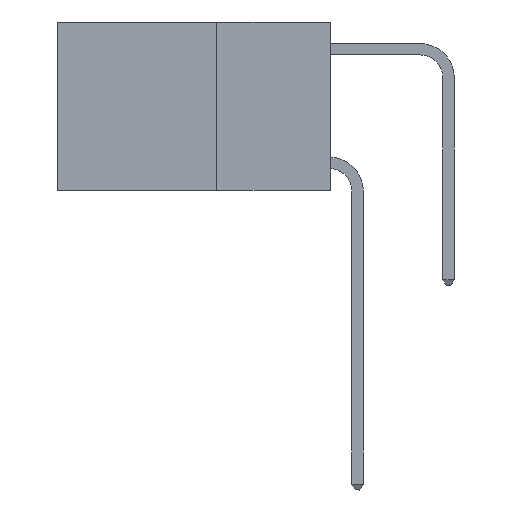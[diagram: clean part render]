
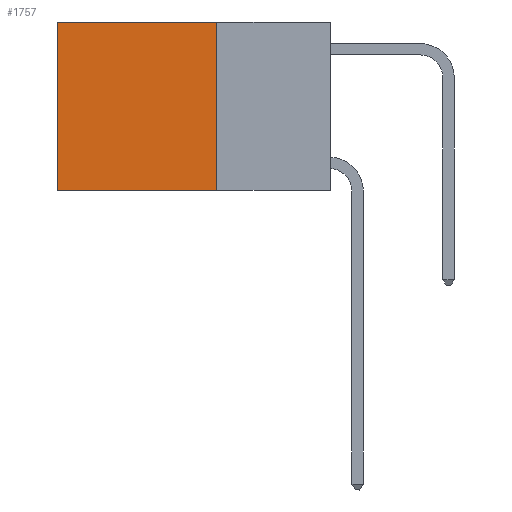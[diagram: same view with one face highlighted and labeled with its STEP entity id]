
A CAD part, left-side view. The second image highlights one B-rep face of the part: STEP entity #1757.
In plain terms, the highlighted planar face has unit normal (-1, 0, 0).
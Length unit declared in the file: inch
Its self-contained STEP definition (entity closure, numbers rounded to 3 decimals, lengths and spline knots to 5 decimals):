
#35 = DIRECTION ( 'NONE',  ( 0., 0., -1. ) ) ;
#761 = CARTESIAN_POINT ( 'NONE',  ( 0.2625, 0.25, 0. ) ) ;
#951 = LINE ( 'NONE', #761, #5265 ) ;
#1168 = LINE ( 'NONE', #11295, #9808 ) ;
#1757 = ADVANCED_FACE ( 'NONE', ( #8471 ), #12451, .F. ) ;
#3666 = EDGE_LOOP ( 'NONE', ( #13763, #18094, #14791, #6608 ) ) ;
#3854 = CARTESIAN_POINT ( 'NONE',  ( 0.2625, 0.6, 0. ) ) ;
#3936 = LINE ( 'NONE', #19762, #6234 ) ;
#4028 = EDGE_CURVE ( 'NONE', #10310, #13068, #17075, .T. ) ;
#5265 = VECTOR ( 'NONE', #12144, 39.37008 ) ;
#6234 = VECTOR ( 'NONE', #11646, 39.37008 ) ;
#6608 = ORIENTED_EDGE ( 'NONE', *, *, #18866, .T. ) ;
#7399 = CARTESIAN_POINT ( 'NONE',  ( 0.2625, 0.25, 0. ) ) ;
#7430 = CARTESIAN_POINT ( 'NONE',  ( 0.2625, 0.25, -0.37 ) ) ;
#8376 = VECTOR ( 'NONE', #19533, 39.37008 ) ;
#8471 = FACE_OUTER_BOUND ( 'NONE', #3666, .T. ) ;
#9048 = AXIS2_PLACEMENT_3D ( 'NONE', #19552, #9784, #35 ) ;
#9784 = DIRECTION ( 'NONE',  ( 1., 0., 0. ) ) ;
#9808 = VECTOR ( 'NONE', #14573, 39.37008 ) ;
#9867 = EDGE_CURVE ( 'NONE', #10169, #15537, #1168, .T. ) ;
#9999 = EDGE_CURVE ( 'NONE', #13068, #15537, #3936, .T. ) ;
#10169 = VERTEX_POINT ( 'NONE', #3854 ) ;
#10310 = VERTEX_POINT ( 'NONE', #7399 ) ;
#11295 = CARTESIAN_POINT ( 'NONE',  ( 0.2625, 0.6, 0. ) ) ;
#11646 = DIRECTION ( 'NONE',  ( 0., 1., 0. ) ) ;
#12144 = DIRECTION ( 'NONE',  ( 0., 1., 0. ) ) ;
#12451 = PLANE ( 'NONE',  #9048 ) ;
#13068 = VERTEX_POINT ( 'NONE', #7430 ) ;
#13763 = ORIENTED_EDGE ( 'NONE', *, *, #9867, .T. ) ;
#14573 = DIRECTION ( 'NONE',  ( 0., 0., -1. ) ) ;
#14791 = ORIENTED_EDGE ( 'NONE', *, *, #4028, .F. ) ;
#15537 = VERTEX_POINT ( 'NONE', #20718 ) ;
#17075 = LINE ( 'NONE', #17873, #8376 ) ;
#17873 = CARTESIAN_POINT ( 'NONE',  ( 0.2625, 0.25, 0. ) ) ;
#18094 = ORIENTED_EDGE ( 'NONE', *, *, #9999, .F. ) ;
#18866 = EDGE_CURVE ( 'NONE', #10310, #10169, #951, .T. ) ;
#19533 = DIRECTION ( 'NONE',  ( 0., 0., -1. ) ) ;
#19552 = CARTESIAN_POINT ( 'NONE',  ( 0.2625, 0.25, 0. ) ) ;
#19762 = CARTESIAN_POINT ( 'NONE',  ( 0.2625, 0.25, -0.37 ) ) ;
#20718 = CARTESIAN_POINT ( 'NONE',  ( 0.2625, 0.6, -0.37 ) ) ;
